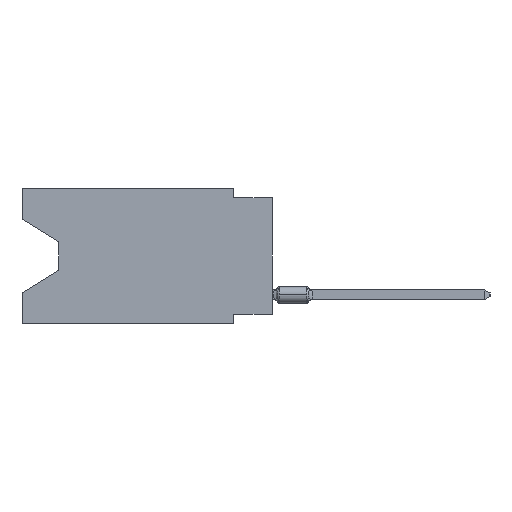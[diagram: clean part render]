
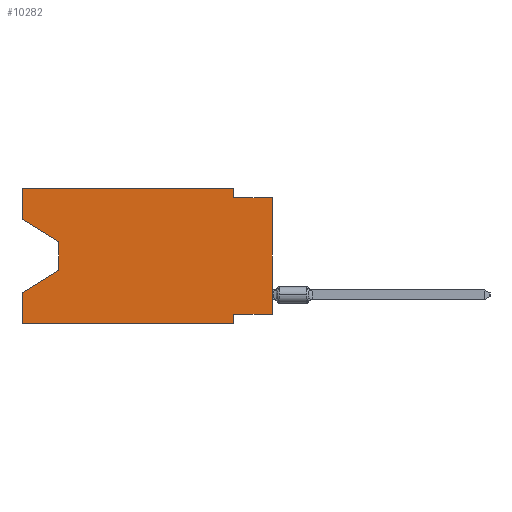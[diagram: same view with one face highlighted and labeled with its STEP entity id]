
A CAD part, left-side view. The second image highlights one B-rep face of the part: STEP entity #10282.
In plain terms, the highlighted planar face has unit normal (-1, 0, 0).
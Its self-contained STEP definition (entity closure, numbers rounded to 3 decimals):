
#75 = CARTESIAN_POINT ( 'NONE',  ( 0., 0., -0.635 ) ) ;
#272 = LINE ( 'NONE', #16414, #2526 ) ;
#866 = EDGE_CURVE ( 'NONE', #26379, #1400, #14266, .T. ) ;
#1400 = VERTEX_POINT ( 'NONE', #46918 ) ;
#1940 = VECTOR ( 'NONE', #41438, 1000. ) ;
#2125 = VECTOR ( 'NONE', #6074, 1000. ) ;
#2332 = EDGE_CURVE ( 'NONE', #22550, #26379, #24265, .T. ) ;
#2526 = VECTOR ( 'NONE', #15894, 1000. ) ;
#3419 = LINE ( 'NONE', #75, #16372 ) ;
#3458 = DIRECTION ( 'NONE',  ( 0., 0., 1. ) ) ;
#4216 = DIRECTION ( 'NONE',  ( 0., 0., -1. ) ) ;
#5461 = DIRECTION ( 'NONE',  ( 0., -1., 0. ) ) ;
#5462 = CARTESIAN_POINT ( 'NONE',  ( 0., 16.383, 0. ) ) ;
#5665 = LINE ( 'NONE', #21284, #44025 ) ;
#6074 = DIRECTION ( 'NONE',  ( 0., 0., 1. ) ) ;
#6172 = ORIENTED_EDGE ( 'NONE', *, *, #41863, .F. ) ;
#6629 = ORIENTED_EDGE ( 'NONE', *, *, #18787, .T. ) ;
#7297 = LINE ( 'NONE', #38568, #31447 ) ;
#7525 = LINE ( 'NONE', #15466, #33626 ) ;
#7816 = DIRECTION ( 'NONE',  ( 0., 1., 0. ) ) ;
#8531 = FACE_OUTER_BOUND ( 'NONE', #30422, .T. ) ;
#10282 = ADVANCED_FACE ( 'NONE', ( #8531 ), #16988, .F. ) ;
#10335 = CARTESIAN_POINT ( 'NONE',  ( 0., 16.383, -2.038 ) ) ;
#10832 = DIRECTION ( 'NONE',  ( 0., -0.855, -0.519 ) ) ;
#11023 = VECTOR ( 'NONE', #36323, 1000. ) ;
#11086 = CARTESIAN_POINT ( 'NONE',  ( 0., 16.383, 0. ) ) ;
#11342 = LINE ( 'NONE', #10335, #30306 ) ;
#11375 = AXIS2_PLACEMENT_3D ( 'NONE', #5462, #43867, #28521 ) ;
#11658 = LINE ( 'NONE', #14987, #23785 ) ;
#12215 = CARTESIAN_POINT ( 'NONE',  ( 0., 13.97, -3.505 ) ) ;
#13730 = VECTOR ( 'NONE', #38009, 1000. ) ;
#13886 = CARTESIAN_POINT ( 'NONE',  ( 0., 2.54, -0.635 ) ) ;
#14266 = LINE ( 'NONE', #29923, #1940 ) ;
#14821 = VERTEX_POINT ( 'NONE', #42802 ) ;
#14987 = CARTESIAN_POINT ( 'NONE',  ( 0., 0., -8.255 ) ) ;
#15466 = CARTESIAN_POINT ( 'NONE',  ( 0., 2.54, -8.89 ) ) ;
#15894 = DIRECTION ( 'NONE',  ( 0., 0., -1. ) ) ;
#16060 = VERTEX_POINT ( 'NONE', #17742 ) ;
#16372 = VECTOR ( 'NONE', #42079, 1000. ) ;
#16414 = CARTESIAN_POINT ( 'NONE',  ( 0., 2.54, 0. ) ) ;
#16677 = CARTESIAN_POINT ( 'NONE',  ( 0., 2.54, 0. ) ) ;
#16988 = PLANE ( 'NONE',  #11375 ) ;
#17081 = EDGE_CURVE ( 'NONE', #36558, #44726, #41898, .T. ) ;
#17742 = CARTESIAN_POINT ( 'NONE',  ( 0., 16.383, -8.89 ) ) ;
#18308 = ORIENTED_EDGE ( 'NONE', *, *, #49309, .F. ) ;
#18787 = EDGE_CURVE ( 'NONE', #16060, #26739, #29024, .T. ) ;
#19171 = VERTEX_POINT ( 'NONE', #16677 ) ;
#20277 = ORIENTED_EDGE ( 'NONE', *, *, #866, .T. ) ;
#21284 = CARTESIAN_POINT ( 'NONE',  ( 0., 16.383, 0. ) ) ;
#21725 = ORIENTED_EDGE ( 'NONE', *, *, #28295, .F. ) ;
#22550 = VERTEX_POINT ( 'NONE', #36149 ) ;
#23056 = VERTEX_POINT ( 'NONE', #41757 ) ;
#23785 = VECTOR ( 'NONE', #7816, 1000. ) ;
#24265 = LINE ( 'NONE', #12215, #11023 ) ;
#24786 = CARTESIAN_POINT ( 'NONE',  ( 0., 13.97, -5.385 ) ) ;
#25081 = EDGE_CURVE ( 'NONE', #40849, #44726, #3419, .T. ) ;
#25345 = EDGE_CURVE ( 'NONE', #14821, #22550, #11342, .T. ) ;
#26379 = VERTEX_POINT ( 'NONE', #24786 ) ;
#26739 = VERTEX_POINT ( 'NONE', #42647 ) ;
#27869 = EDGE_CURVE ( 'NONE', #36558, #23056, #11658, .T. ) ;
#28295 = EDGE_CURVE ( 'NONE', #19171, #40849, #272, .T. ) ;
#28521 = DIRECTION ( 'NONE',  ( 0., 0., -1. ) ) ;
#29024 = LINE ( 'NONE', #33131, #40563 ) ;
#29506 = ORIENTED_EDGE ( 'NONE', *, *, #39715, .F. ) ;
#29923 = CARTESIAN_POINT ( 'NONE',  ( 0., 13.97, -5.385 ) ) ;
#30306 = VECTOR ( 'NONE', #10832, 1000. ) ;
#30422 = EDGE_LOOP ( 'NONE', ( #35785, #35664, #20277, #30917, #6629, #6172, #32271, #49659, #47421, #21725, #29506, #18308 ) ) ;
#30917 = ORIENTED_EDGE ( 'NONE', *, *, #37204, .F. ) ;
#31447 = VECTOR ( 'NONE', #3458, 1000. ) ;
#32271 = ORIENTED_EDGE ( 'NONE', *, *, #27869, .F. ) ;
#33131 = CARTESIAN_POINT ( 'NONE',  ( 0., 16.383, -8.89 ) ) ;
#33330 = DIRECTION ( 'NONE',  ( 0., 0., 1. ) ) ;
#33626 = VECTOR ( 'NONE', #4216, 1000. ) ;
#35664 = ORIENTED_EDGE ( 'NONE', *, *, #2332, .T. ) ;
#35785 = ORIENTED_EDGE ( 'NONE', *, *, #25345, .T. ) ;
#36149 = CARTESIAN_POINT ( 'NONE',  ( 0., 13.97, -3.505 ) ) ;
#36323 = DIRECTION ( 'NONE',  ( 0., 0., -1. ) ) ;
#36558 = VERTEX_POINT ( 'NONE', #43625 ) ;
#37204 = EDGE_CURVE ( 'NONE', #16060, #1400, #5665, .T. ) ;
#37853 = CARTESIAN_POINT ( 'NONE',  ( 0., 0., -0.635 ) ) ;
#38009 = DIRECTION ( 'NONE',  ( 0., -1., 0. ) ) ;
#38568 = CARTESIAN_POINT ( 'NONE',  ( 0., 16.383, 0. ) ) ;
#38861 = CARTESIAN_POINT ( 'NONE',  ( 0., 16.383, 0. ) ) ;
#39715 = EDGE_CURVE ( 'NONE', #44941, #19171, #49729, .T. ) ;
#40563 = VECTOR ( 'NONE', #5461, 1000. ) ;
#40849 = VERTEX_POINT ( 'NONE', #13886 ) ;
#41438 = DIRECTION ( 'NONE',  ( 0., 0.855, -0.519 ) ) ;
#41757 = CARTESIAN_POINT ( 'NONE',  ( 0., 2.54, -8.255 ) ) ;
#41863 = EDGE_CURVE ( 'NONE', #23056, #26739, #7525, .T. ) ;
#41898 = LINE ( 'NONE', #45493, #2125 ) ;
#42079 = DIRECTION ( 'NONE',  ( 0., -1., 0. ) ) ;
#42647 = CARTESIAN_POINT ( 'NONE',  ( 0., 2.54, -8.89 ) ) ;
#42802 = CARTESIAN_POINT ( 'NONE',  ( 0., 16.383, -2.038 ) ) ;
#43625 = CARTESIAN_POINT ( 'NONE',  ( 0., 0., -8.255 ) ) ;
#43867 = DIRECTION ( 'NONE',  ( 1., 0., 0. ) ) ;
#44025 = VECTOR ( 'NONE', #33330, 1000. ) ;
#44726 = VERTEX_POINT ( 'NONE', #37853 ) ;
#44941 = VERTEX_POINT ( 'NONE', #38861 ) ;
#45493 = CARTESIAN_POINT ( 'NONE',  ( 0., 0., 0. ) ) ;
#46918 = CARTESIAN_POINT ( 'NONE',  ( 0., 16.383, -6.852 ) ) ;
#47421 = ORIENTED_EDGE ( 'NONE', *, *, #25081, .F. ) ;
#49309 = EDGE_CURVE ( 'NONE', #14821, #44941, #7297, .T. ) ;
#49659 = ORIENTED_EDGE ( 'NONE', *, *, #17081, .T. ) ;
#49729 = LINE ( 'NONE', #11086, #13730 ) ;
